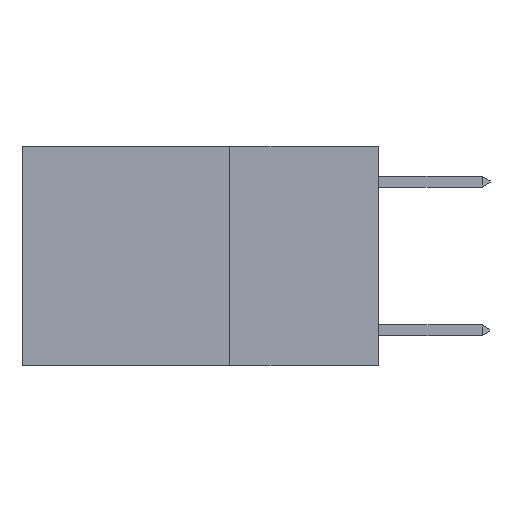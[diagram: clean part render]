
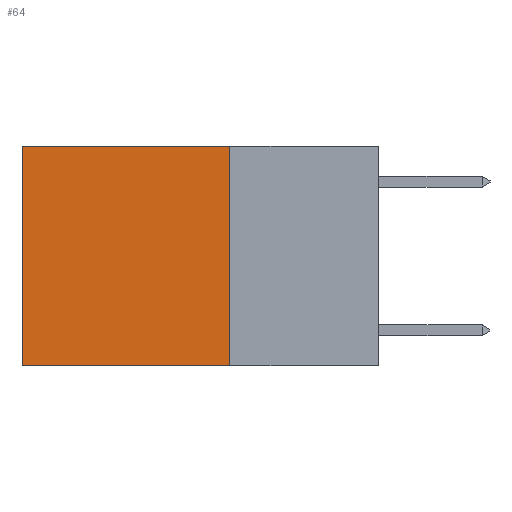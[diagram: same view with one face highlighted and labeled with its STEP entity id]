
A CAD part, left-side view. The second image highlights one B-rep face of the part: STEP entity #64.
In plain terms, the highlighted planar face has unit normal (-1, 0, 0).
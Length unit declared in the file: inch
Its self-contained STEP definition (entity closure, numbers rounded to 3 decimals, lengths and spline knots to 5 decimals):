
#64 = ADVANCED_FACE ( 'NONE', ( #4019 ), #2877, .F. ) ;
#259 = VERTEX_POINT ( 'NONE', #4670 ) ;
#1027 = DIRECTION ( 'NONE',  ( 1., 0., 0. ) ) ;
#1091 = DIRECTION ( 'NONE',  ( 0., 0., -1. ) ) ;
#1202 = DIRECTION ( 'NONE',  ( 0., 1., 0. ) ) ;
#1315 = EDGE_CURVE ( 'NONE', #4309, #6840, #4098, .T. ) ;
#1349 = DIRECTION ( 'NONE',  ( 0., 0., -1. ) ) ;
#1853 = EDGE_LOOP ( 'NONE', ( #8165, #2512, #2521, #5616 ) ) ;
#1871 = CARTESIAN_POINT ( 'NONE',  ( 0.2625, 0.25, -0.37 ) ) ;
#2512 = ORIENTED_EDGE ( 'NONE', *, *, #4422, .F. ) ;
#2521 = ORIENTED_EDGE ( 'NONE', *, *, #7861, .F. ) ;
#2877 = PLANE ( 'NONE',  #7258 ) ;
#3127 = CARTESIAN_POINT ( 'NONE',  ( 0.2625, 0.25, 0. ) ) ;
#3427 = EDGE_CURVE ( 'NONE', #6840, #6727, #3981, .T. ) ;
#3896 = VECTOR ( 'NONE', #1349, 39.37008 ) ;
#3912 = VECTOR ( 'NONE', #7694, 39.37008 ) ;
#3973 = VECTOR ( 'NONE', #8217, 39.37008 ) ;
#3981 = LINE ( 'NONE', #5897, #3973 ) ;
#4019 = FACE_OUTER_BOUND ( 'NONE', #1853, .T. ) ;
#4098 = LINE ( 'NONE', #5963, #3912 ) ;
#4309 = VERTEX_POINT ( 'NONE', #5202 ) ;
#4357 = LINE ( 'NONE', #4613, #3896 ) ;
#4422 = EDGE_CURVE ( 'NONE', #259, #6727, #7931, .T. ) ;
#4613 = CARTESIAN_POINT ( 'NONE',  ( 0.2625, 0.25, 0. ) ) ;
#4670 = CARTESIAN_POINT ( 'NONE',  ( 0.2625, 0.25, -0.37 ) ) ;
#5202 = CARTESIAN_POINT ( 'NONE',  ( 0.2625, 0.25, 0. ) ) ;
#5616 = ORIENTED_EDGE ( 'NONE', *, *, #1315, .T. ) ;
#5897 = CARTESIAN_POINT ( 'NONE',  ( 0.2625, 0.6, 0. ) ) ;
#5963 = CARTESIAN_POINT ( 'NONE',  ( 0.2625, 0.25, 0. ) ) ;
#6727 = VERTEX_POINT ( 'NONE', #7718 ) ;
#6840 = VERTEX_POINT ( 'NONE', #7242 ) ;
#7242 = CARTESIAN_POINT ( 'NONE',  ( 0.2625, 0.6, 0. ) ) ;
#7258 = AXIS2_PLACEMENT_3D ( 'NONE', #3127, #1027, #1091 ) ;
#7632 = VECTOR ( 'NONE', #1202, 39.37008 ) ;
#7694 = DIRECTION ( 'NONE',  ( 0., 1., 0. ) ) ;
#7718 = CARTESIAN_POINT ( 'NONE',  ( 0.2625, 0.6, -0.37 ) ) ;
#7861 = EDGE_CURVE ( 'NONE', #4309, #259, #4357, .T. ) ;
#7931 = LINE ( 'NONE', #1871, #7632 ) ;
#8165 = ORIENTED_EDGE ( 'NONE', *, *, #3427, .T. ) ;
#8217 = DIRECTION ( 'NONE',  ( 0., 0., -1. ) ) ;
